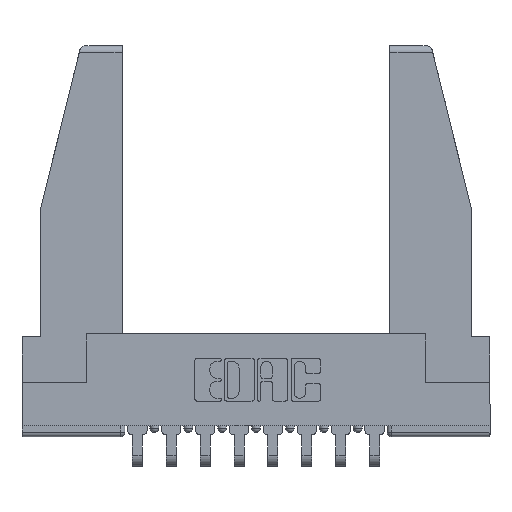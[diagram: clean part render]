
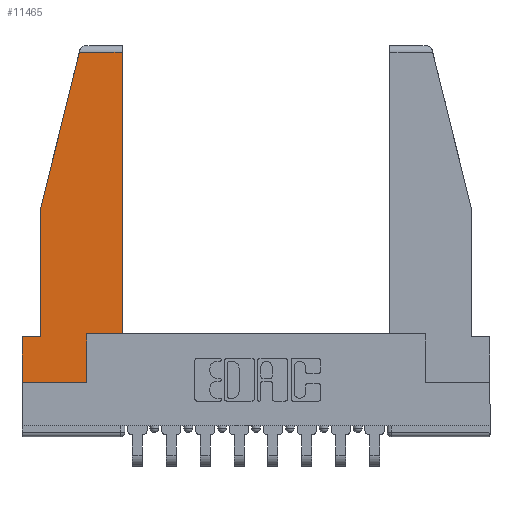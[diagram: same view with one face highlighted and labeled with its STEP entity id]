
A CAD part, top view. The second image highlights one B-rep face of the part: STEP entity #11465.
In plain terms, the highlighted planar face has unit normal (0, 0, 1).
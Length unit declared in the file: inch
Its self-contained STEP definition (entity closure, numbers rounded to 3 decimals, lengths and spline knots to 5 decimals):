
#91 = CARTESIAN_POINT ( 'NONE',  ( 0.086, 0.21, 0. ) ) ;
#284 = CARTESIAN_POINT ( 'NONE',  ( 0.271, 1.55, 0. ) ) ;
#395 = DIRECTION ( 'NONE',  ( -1., 0., 0. ) ) ;
#617 = ORIENTED_EDGE ( 'NONE', *, *, #11993, .T. ) ;
#684 = ORIENTED_EDGE ( 'NONE', *, *, #5176, .T. ) ;
#812 = VERTEX_POINT ( 'NONE', #13409 ) ;
#891 = EDGE_CURVE ( 'NONE', #1207, #3025, #12120, .T. ) ;
#1099 = CARTESIAN_POINT ( 'NONE',  ( 0.297, 0.223, 0. ) ) ;
#1207 = VERTEX_POINT ( 'NONE', #1437 ) ;
#1267 = FACE_OUTER_BOUND ( 'NONE', #11074, .T. ) ;
#1437 = CARTESIAN_POINT ( 'NONE',  ( 0.461, 0.223, 0. ) ) ;
#1582 = CARTESIAN_POINT ( 'NONE',  ( 0.461, 1.52, 0. ) ) ;
#1785 = VECTOR ( 'NONE', #11483, 39.37008 ) ;
#2395 = VECTOR ( 'NONE', #10550, 39.37008 ) ;
#3025 = VERTEX_POINT ( 'NONE', #1582 ) ;
#3065 = LINE ( 'NONE', #7608, #13584 ) ;
#3095 = VERTEX_POINT ( 'NONE', #7102 ) ;
#3247 = CARTESIAN_POINT ( 'NONE',  ( 0., 0., 0. ) ) ;
#3429 = VERTEX_POINT ( 'NONE', #91 ) ;
#3559 = PLANE ( 'NONE',  #12843 ) ;
#4107 = EDGE_CURVE ( 'NONE', #7830, #4775, #10842, .T. ) ;
#4145 = VECTOR ( 'NONE', #395, 39.37008 ) ;
#4195 = EDGE_CURVE ( 'NONE', #3025, #3095, #7401, .T. ) ;
#4441 = DIRECTION ( 'NONE',  ( 0., -1., 0. ) ) ;
#4720 = DIRECTION ( 'NONE',  ( 1., 0., 0. ) ) ;
#4775 = VERTEX_POINT ( 'NONE', #1099 ) ;
#4844 = ORIENTED_EDGE ( 'NONE', *, *, #11446, .T. ) ;
#5075 = VECTOR ( 'NONE', #6122, 39.37008 ) ;
#5176 = EDGE_CURVE ( 'NONE', #812, #6077, #6082, .T. ) ;
#5571 = EDGE_CURVE ( 'NONE', #13398, #3429, #3065, .T. ) ;
#5901 = VECTOR ( 'NONE', #8821, 39.37008 ) ;
#6077 = VERTEX_POINT ( 'NONE', #3247 ) ;
#6082 = LINE ( 'NONE', #7030, #5075 ) ;
#6122 = DIRECTION ( 'NONE',  ( 0., -1., 0. ) ) ;
#7030 = CARTESIAN_POINT ( 'NONE',  ( 0., 0.21, 0. ) ) ;
#7102 = CARTESIAN_POINT ( 'NONE',  ( 0.2636, 1.52, 0. ) ) ;
#7178 = LINE ( 'NONE', #9621, #12914 ) ;
#7401 = LINE ( 'NONE', #13486, #1785 ) ;
#7428 = LINE ( 'NONE', #8877, #8443 ) ;
#7608 = CARTESIAN_POINT ( 'NONE',  ( 0.086, 0.8, 0. ) ) ;
#7830 = VERTEX_POINT ( 'NONE', #11625 ) ;
#8061 = CARTESIAN_POINT ( 'NONE',  ( 0.297, 0., 0. ) ) ;
#8101 = EDGE_CURVE ( 'NONE', #3429, #812, #10388, .T. ) ;
#8146 = EDGE_CURVE ( 'NONE', #4775, #1207, #7428, .T. ) ;
#8332 = CARTESIAN_POINT ( 'NONE',  ( 0.461, 0.223, 0. ) ) ;
#8443 = VECTOR ( 'NONE', #12978, 39.37008 ) ;
#8496 = ORIENTED_EDGE ( 'NONE', *, *, #5571, .T. ) ;
#8584 = ORIENTED_EDGE ( 'NONE', *, *, #8101, .T. ) ;
#8793 = CARTESIAN_POINT ( 'NONE',  ( 0., 0.21, 0. ) ) ;
#8821 = DIRECTION ( 'NONE',  ( -0.239, -0.971, 0. ) ) ;
#8877 = CARTESIAN_POINT ( 'NONE',  ( 0.297, 0.223, 0. ) ) ;
#9320 = LINE ( 'NONE', #284, #5901 ) ;
#9367 = DIRECTION ( 'NONE',  ( 0., 1., 0. ) ) ;
#9621 = CARTESIAN_POINT ( 'NONE',  ( 0., 0., 0. ) ) ;
#9940 = CARTESIAN_POINT ( 'NONE',  ( 0., 0., 0. ) ) ;
#10388 = LINE ( 'NONE', #8793, #4145 ) ;
#10533 = CARTESIAN_POINT ( 'NONE',  ( 0.086, 0.8, 0. ) ) ;
#10550 = DIRECTION ( 'NONE',  ( 0., 1., 0. ) ) ;
#10794 = ORIENTED_EDGE ( 'NONE', *, *, #4107, .T. ) ;
#10842 = LINE ( 'NONE', #8061, #11833 ) ;
#10992 = DIRECTION ( 'NONE',  ( 0., 0., 1. ) ) ;
#11074 = EDGE_LOOP ( 'NONE', ( #12785, #12060, #4844, #8496, #8584, #684, #617, #10794, #13267 ) ) ;
#11446 = EDGE_CURVE ( 'NONE', #3095, #13398, #9320, .T. ) ;
#11465 = ADVANCED_FACE ( 'NONE', ( #1267 ), #3559, .T. ) ;
#11483 = DIRECTION ( 'NONE',  ( -1., 0., 0. ) ) ;
#11625 = CARTESIAN_POINT ( 'NONE',  ( 0.297, 0., 0. ) ) ;
#11833 = VECTOR ( 'NONE', #9367, 39.37008 ) ;
#11993 = EDGE_CURVE ( 'NONE', #6077, #7830, #7178, .T. ) ;
#12060 = ORIENTED_EDGE ( 'NONE', *, *, #4195, .T. ) ;
#12120 = LINE ( 'NONE', #8332, #2395 ) ;
#12737 = DIRECTION ( 'NONE',  ( 1., 0., 0. ) ) ;
#12785 = ORIENTED_EDGE ( 'NONE', *, *, #891, .T. ) ;
#12843 = AXIS2_PLACEMENT_3D ( 'NONE', #9940, #10992, #4720 ) ;
#12914 = VECTOR ( 'NONE', #12737, 39.37008 ) ;
#12978 = DIRECTION ( 'NONE',  ( 1., 0., 0. ) ) ;
#13267 = ORIENTED_EDGE ( 'NONE', *, *, #8146, .T. ) ;
#13398 = VERTEX_POINT ( 'NONE', #10533 ) ;
#13409 = CARTESIAN_POINT ( 'NONE',  ( 0., 0.21, 0. ) ) ;
#13486 = CARTESIAN_POINT ( 'NONE',  ( 0., 1.52, 0. ) ) ;
#13584 = VECTOR ( 'NONE', #4441, 39.37008 ) ;
